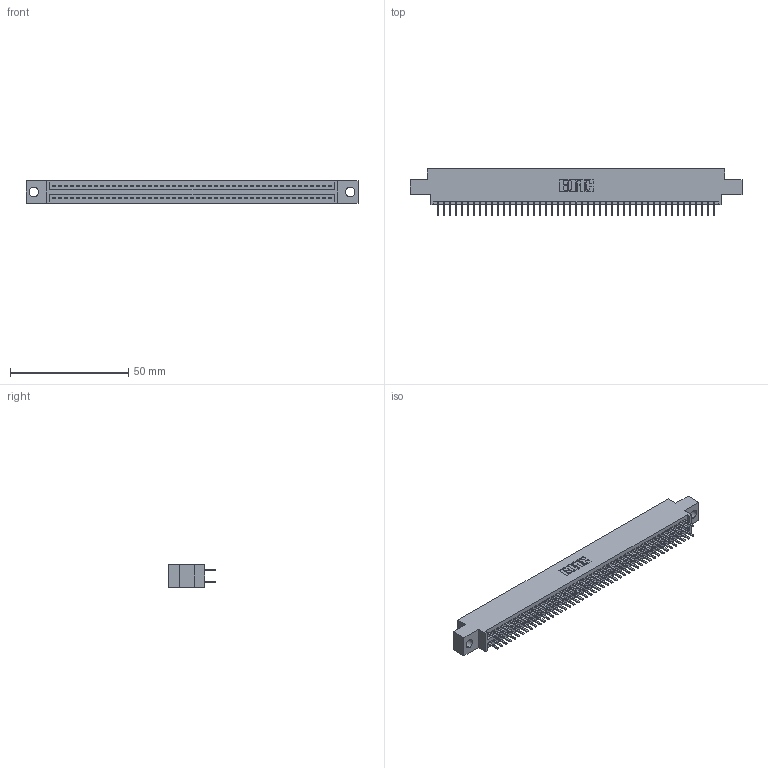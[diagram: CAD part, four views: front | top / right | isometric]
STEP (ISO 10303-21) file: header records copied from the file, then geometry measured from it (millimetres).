
FILE_DESCRIPTION (( 'STEP AP203' ), '1' );
FILE_NAME ('345-094-520-804.STEP', '2018-10-04T23:32:22', ( '' ), ( '' ), 'SwSTEP 2.0', 'SolidWorks 2016', '' );
FILE_SCHEMA (( 'CONFIG_CONTROL_DESIGN' ));
Length unit declared in the file: inch
Products named in the file (3): 345-094-520-804; 345 Part_0.170 Offset - 0.156 Dia-TH; 345-292-001_345-293-120
Assembly tree (95 placements, depth 2):
  345-094-520-804
    345 Part_0.170 Offset - 0.156 Dia-TH
    345-292-001_345-293-120  x94
Bounding box: 140.59 x 19.68 x 9.4 mm (x, y, z)
Volume: 13460.8 mm3; surface area: 19864.9 mm2
Topology: 95 solids, 95 shells, 5206 faces, 15111 edges, 9822 vertices
Faces by surface type: plane 3374, cylinder 1832
Entity records: 36453 total; most frequent: CARTESIAN_POINT 6120, ORIENTED_EDGE 6042, DIRECTION 5377, EDGE_CURVE 3021, VECTOR 2697, LINE 2697, VERTEX_POINT 2010, AXIS2_PLACEMENT_3D 1340
